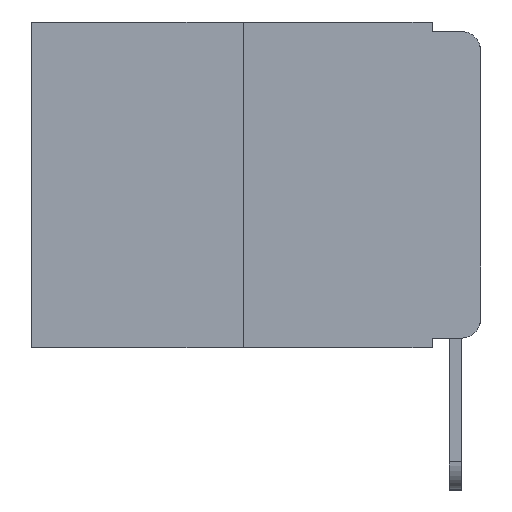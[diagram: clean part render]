
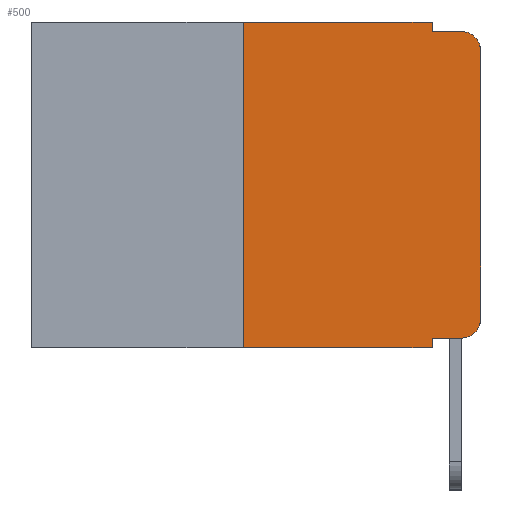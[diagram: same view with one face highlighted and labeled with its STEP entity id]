
A CAD part, left-side view. The second image highlights one B-rep face of the part: STEP entity #500.
In plain terms, the highlighted planar face has unit normal (-1, 0, 0).
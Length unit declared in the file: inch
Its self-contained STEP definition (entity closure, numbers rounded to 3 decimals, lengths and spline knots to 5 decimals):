
#14 = PLANE ( 'NONE',  #7230 ) ;
#200 = VERTEX_POINT ( 'NONE', #6719 ) ;
#201 = ORIENTED_EDGE ( 'NONE', *, *, #2083, .T. ) ;
#263 = EDGE_LOOP ( 'NONE', ( #201, #592, #738, #1259, #1371, #2622, #6348, #7530, #7711, #9616 ) ) ;
#500 = ADVANCED_FACE ( 'NONE', ( #12578 ), #14, .F. ) ;
#592 = ORIENTED_EDGE ( 'NONE', *, *, #2126, .T. ) ;
#672 = VERTEX_POINT ( 'NONE', #12752 ) ;
#738 = ORIENTED_EDGE ( 'NONE', *, *, #2146, .F. ) ;
#914 = CARTESIAN_POINT ( 'NONE',  ( 0., 0.051, -0.333 ) ) ;
#1259 = ORIENTED_EDGE ( 'NONE', *, *, #2168, .F. ) ;
#1371 = ORIENTED_EDGE ( 'NONE', *, *, #1754, .F. ) ;
#1466 = LINE ( 'NONE', #13118, #9851 ) ;
#1575 = AXIS2_PLACEMENT_3D ( 'NONE', #12733, #6782, #13667 ) ;
#1718 = DIRECTION ( 'NONE',  ( 0., 0., -1. ) ) ;
#1754 = EDGE_CURVE ( 'NONE', #672, #8487, #8136, .T. ) ;
#1826 = CARTESIAN_POINT ( 'NONE',  ( 0., 0.02, -0.333 ) ) ;
#1921 = CARTESIAN_POINT ( 'NONE',  ( 0., 0.473, 0. ) ) ;
#2083 = EDGE_CURVE ( 'NONE', #2966, #13323, #13292, .T. ) ;
#2090 = LINE ( 'NONE', #13373, #9707 ) ;
#2126 = EDGE_CURVE ( 'NONE', #13323, #9199, #8121, .T. ) ;
#2146 = EDGE_CURVE ( 'NONE', #200, #9199, #7791, .T. ) ;
#2168 = EDGE_CURVE ( 'NONE', #8487, #200, #1466, .T. ) ;
#2188 = EDGE_CURVE ( 'NONE', #12805, #672, #12376, .T. ) ;
#2190 = EDGE_CURVE ( 'NONE', #10197, #8746, #9223, .T. ) ;
#2253 = VERTEX_POINT ( 'NONE', #1826 ) ;
#2415 = EDGE_CURVE ( 'NONE', #10197, #2253, #4442, .T. ) ;
#2453 = CARTESIAN_POINT ( 'NONE',  ( 0., 0., -0.03 ) ) ;
#2508 = EDGE_CURVE ( 'NONE', #2253, #2966, #5952, .T. ) ;
#2578 = VECTOR ( 'NONE', #1718, 39.37008 ) ;
#2622 = ORIENTED_EDGE ( 'NONE', *, *, #2188, .F. ) ;
#2901 = DIRECTION ( 'NONE',  ( 0., -1., 0. ) ) ;
#2966 = VERTEX_POINT ( 'NONE', #13101 ) ;
#3825 = DIRECTION ( 'NONE',  ( -1., 0., 0. ) ) ;
#3867 = AXIS2_PLACEMENT_3D ( 'NONE', #10153, #3825, #11148 ) ;
#4043 = DIRECTION ( 'NONE',  ( 0., 0., 1. ) ) ;
#4442 = LINE ( 'NONE', #914, #6944 ) ;
#4962 = VECTOR ( 'NONE', #8196, 39.37008 ) ;
#5333 = CARTESIAN_POINT ( 'NONE',  ( 0., 0.25, -0.343 ) ) ;
#5403 = CARTESIAN_POINT ( 'NONE',  ( 0., 0.02, -0.01 ) ) ;
#5952 = CIRCLE ( 'NONE', #1575, 0.02 ) ;
#6348 = ORIENTED_EDGE ( 'NONE', *, *, #10504, .T. ) ;
#6719 = CARTESIAN_POINT ( 'NONE',  ( 0., 0.051, -0.01 ) ) ;
#6782 = DIRECTION ( 'NONE',  ( -1., 0., 0. ) ) ;
#6944 = VECTOR ( 'NONE', #7690, 39.37008 ) ;
#7104 = CARTESIAN_POINT ( 'NONE',  ( 0., 0.051, -0.333 ) ) ;
#7221 = DIRECTION ( 'NONE',  ( 0., 0., -1. ) ) ;
#7230 = AXIS2_PLACEMENT_3D ( 'NONE', #1921, #13739, #7856 ) ;
#7530 = ORIENTED_EDGE ( 'NONE', *, *, #2190, .F. ) ;
#7564 = DIRECTION ( 'NONE',  ( 0., -1., 0. ) ) ;
#7690 = DIRECTION ( 'NONE',  ( 0., -1., 0. ) ) ;
#7711 = ORIENTED_EDGE ( 'NONE', *, *, #2415, .T. ) ;
#7791 = LINE ( 'NONE', #13039, #4962 ) ;
#7856 = DIRECTION ( 'NONE',  ( 0., 0., -1. ) ) ;
#8054 = CARTESIAN_POINT ( 'NONE',  ( 0., 0., 0. ) ) ;
#8121 = CIRCLE ( 'NONE', #3867, 0.02 ) ;
#8136 = LINE ( 'NONE', #9398, #8479 ) ;
#8196 = DIRECTION ( 'NONE',  ( 0., -1., 0. ) ) ;
#8382 = CARTESIAN_POINT ( 'NONE',  ( 0., 0.051, 0. ) ) ;
#8479 = VECTOR ( 'NONE', #2901, 39.37008 ) ;
#8487 = VERTEX_POINT ( 'NONE', #12454 ) ;
#8746 = VERTEX_POINT ( 'NONE', #10400 ) ;
#9199 = VERTEX_POINT ( 'NONE', #5403 ) ;
#9223 = LINE ( 'NONE', #8382, #2578 ) ;
#9342 = CARTESIAN_POINT ( 'NONE',  ( 0., 0.25, 0. ) ) ;
#9398 = CARTESIAN_POINT ( 'NONE',  ( 0., 0.473, 0. ) ) ;
#9536 = VECTOR ( 'NONE', #4043, 39.37008 ) ;
#9616 = ORIENTED_EDGE ( 'NONE', *, *, #2508, .T. ) ;
#9707 = VECTOR ( 'NONE', #7564, 39.37008 ) ;
#9851 = VECTOR ( 'NONE', #7221, 39.37008 ) ;
#10153 = CARTESIAN_POINT ( 'NONE',  ( 0., 0.02, -0.03 ) ) ;
#10197 = VERTEX_POINT ( 'NONE', #7104 ) ;
#10400 = CARTESIAN_POINT ( 'NONE',  ( 0., 0.051, -0.343 ) ) ;
#10504 = EDGE_CURVE ( 'NONE', #12805, #8746, #2090, .T. ) ;
#10757 = VECTOR ( 'NONE', #11060, 39.37008 ) ;
#11060 = DIRECTION ( 'NONE',  ( 0., 0., 1. ) ) ;
#11148 = DIRECTION ( 'NONE',  ( 0., 0., -1. ) ) ;
#12376 = LINE ( 'NONE', #9342, #9536 ) ;
#12454 = CARTESIAN_POINT ( 'NONE',  ( 0., 0.051, 0. ) ) ;
#12578 = FACE_OUTER_BOUND ( 'NONE', #263, .T. ) ;
#12733 = CARTESIAN_POINT ( 'NONE',  ( 0., 0.02, -0.313 ) ) ;
#12752 = CARTESIAN_POINT ( 'NONE',  ( 0., 0.25, 0. ) ) ;
#12805 = VERTEX_POINT ( 'NONE', #5333 ) ;
#13039 = CARTESIAN_POINT ( 'NONE',  ( 0., 0.051, -0.01 ) ) ;
#13101 = CARTESIAN_POINT ( 'NONE',  ( 0., 0., -0.313 ) ) ;
#13118 = CARTESIAN_POINT ( 'NONE',  ( 0., 0.051, 0. ) ) ;
#13292 = LINE ( 'NONE', #8054, #10757 ) ;
#13323 = VERTEX_POINT ( 'NONE', #2453 ) ;
#13373 = CARTESIAN_POINT ( 'NONE',  ( 0., 0.473, -0.343 ) ) ;
#13667 = DIRECTION ( 'NONE',  ( 0., 0., -1. ) ) ;
#13739 = DIRECTION ( 'NONE',  ( 1., 0., 0. ) ) ;
